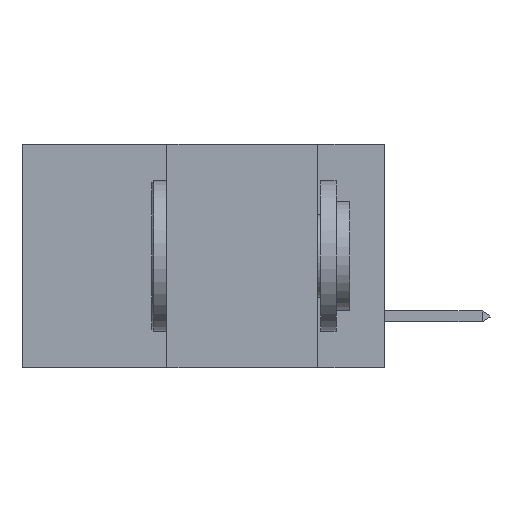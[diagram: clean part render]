
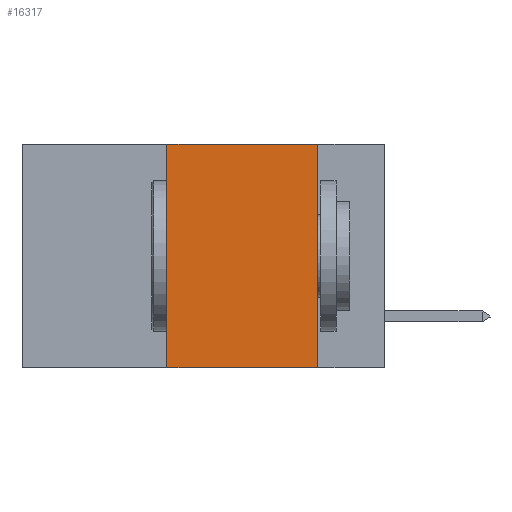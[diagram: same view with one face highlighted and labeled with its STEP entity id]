
A CAD part, left-side view. The second image highlights one B-rep face of the part: STEP entity #16317.
In plain terms, the highlighted planar face has unit normal (-1, 0, 0).
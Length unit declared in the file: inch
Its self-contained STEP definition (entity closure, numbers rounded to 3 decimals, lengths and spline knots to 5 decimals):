
#510 = CARTESIAN_POINT ( 'NONE',  ( 0., 0.11, 0. ) ) ;
#2472 = EDGE_CURVE ( 'NONE', #12178, #34998, #12534, .T. ) ;
#4827 = VECTOR ( 'NONE', #31347, 39.37008 ) ;
#7313 = FACE_OUTER_BOUND ( 'NONE', #34861, .T. ) ;
#11795 = LINE ( 'NONE', #510, #4827 ) ;
#12178 = VERTEX_POINT ( 'NONE', #37513 ) ;
#12498 = CARTESIAN_POINT ( 'NONE',  ( 0., 0.36, 0. ) ) ;
#12534 = LINE ( 'NONE', #38079, #27584 ) ;
#12970 = CARTESIAN_POINT ( 'NONE',  ( 0., 0.36, -0.37 ) ) ;
#14304 = VECTOR ( 'NONE', #42969, 39.37008 ) ;
#14709 = ORIENTED_EDGE ( 'NONE', *, *, #43834, .F. ) ;
#15369 = VERTEX_POINT ( 'NONE', #42093 ) ;
#15898 = LINE ( 'NONE', #12498, #14304 ) ;
#16317 = ADVANCED_FACE ( 'NONE', ( #7313 ), #19255, .F. ) ;
#16352 = VECTOR ( 'NONE', #34827, 39.37008 ) ;
#17593 = CARTESIAN_POINT ( 'NONE',  ( 0., 0.6, -0.37 ) ) ;
#19255 = PLANE ( 'NONE',  #36887 ) ;
#19974 = ORIENTED_EDGE ( 'NONE', *, *, #28008, .F. ) ;
#21171 = DIRECTION ( 'NONE',  ( 0., -1., 0. ) ) ;
#26372 = DIRECTION ( 'NONE',  ( 1., 0., 0. ) ) ;
#27584 = VECTOR ( 'NONE', #21171, 39.37008 ) ;
#28008 = EDGE_CURVE ( 'NONE', #34998, #15369, #11795, .T. ) ;
#28519 = VERTEX_POINT ( 'NONE', #12970 ) ;
#31347 = DIRECTION ( 'NONE',  ( 0., 0., -1. ) ) ;
#32357 = ORIENTED_EDGE ( 'NONE', *, *, #36094, .T. ) ;
#34827 = DIRECTION ( 'NONE',  ( 0., -1., 0. ) ) ;
#34861 = EDGE_LOOP ( 'NONE', ( #19974, #44101, #14709, #32357 ) ) ;
#34998 = VERTEX_POINT ( 'NONE', #40445 ) ;
#36094 = EDGE_CURVE ( 'NONE', #28519, #15369, #38255, .T. ) ;
#36471 = DIRECTION ( 'NONE',  ( 0., 0., -1. ) ) ;
#36887 = AXIS2_PLACEMENT_3D ( 'NONE', #43707, #26372, #36471 ) ;
#37513 = CARTESIAN_POINT ( 'NONE',  ( 0., 0.36, 0. ) ) ;
#38079 = CARTESIAN_POINT ( 'NONE',  ( 0., 0.6, 0. ) ) ;
#38255 = LINE ( 'NONE', #17593, #16352 ) ;
#40445 = CARTESIAN_POINT ( 'NONE',  ( 0., 0.11, 0. ) ) ;
#42093 = CARTESIAN_POINT ( 'NONE',  ( 0., 0.11, -0.37 ) ) ;
#42969 = DIRECTION ( 'NONE',  ( 0., 0., 1. ) ) ;
#43707 = CARTESIAN_POINT ( 'NONE',  ( 0., 0.6, 0. ) ) ;
#43834 = EDGE_CURVE ( 'NONE', #28519, #12178, #15898, .T. ) ;
#44101 = ORIENTED_EDGE ( 'NONE', *, *, #2472, .F. ) ;
